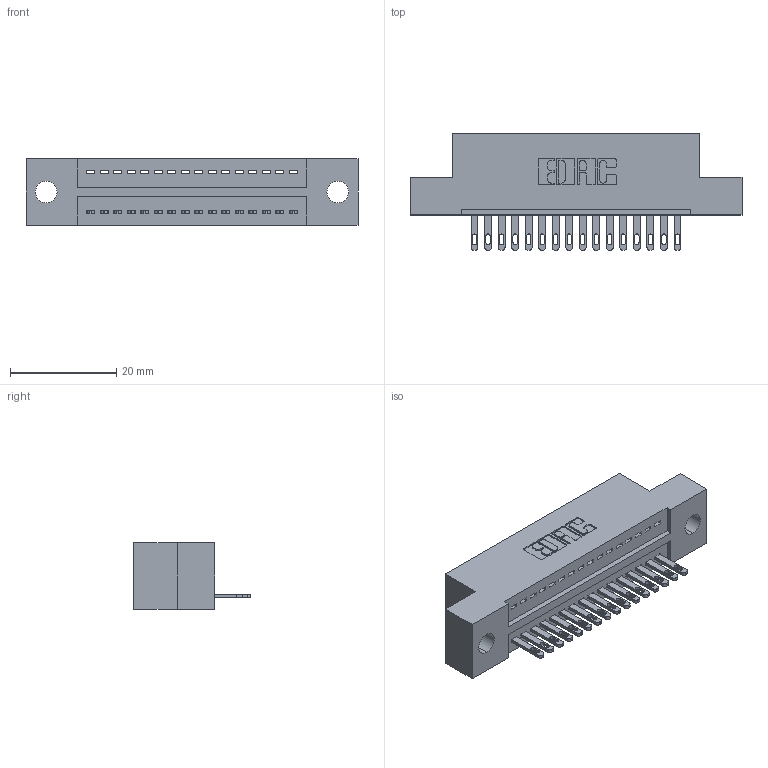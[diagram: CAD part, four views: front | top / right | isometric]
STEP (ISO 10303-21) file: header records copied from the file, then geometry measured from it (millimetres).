
FILE_DESCRIPTION (( 'STEP AP203' ), '1' );
FILE_NAME ('325-016-500-109.STEP', '2020-02-24T16:09:55', ( '' ), ( '' ), 'SwSTEP 2.0', 'SolidWorks 2016', '' );
FILE_SCHEMA (( 'CONFIG_CONTROL_DESIGN' ));
Length unit declared in the file: inch
Products named in the file (3): 325 Part_.160 TH; 325-292-001_325-293-100; 325-016-500-109
Assembly tree (17 placements, depth 2):
  325-016-500-109
    325 Part_.160 TH
    325-292-001_325-293-100  x16
Bounding box: 62.36 x 21.84 x 12.45 mm (x, y, z)
Volume: 7490.9 mm3; surface area: 7676 mm2
Topology: 17 solids, 17 shells, 978 faces, 2999 edges, 1998 vertices
Faces by surface type: plane 646, cylinder 332
Entity records: 13077 total; most frequent: CARTESIAN_POINT 2266, ORIENTED_EDGE 2218, DIRECTION 1965, EDGE_CURVE 1109, LINE 977, VECTOR 977, VERTEX_POINT 738, AXIS2_PLACEMENT_3D 494
